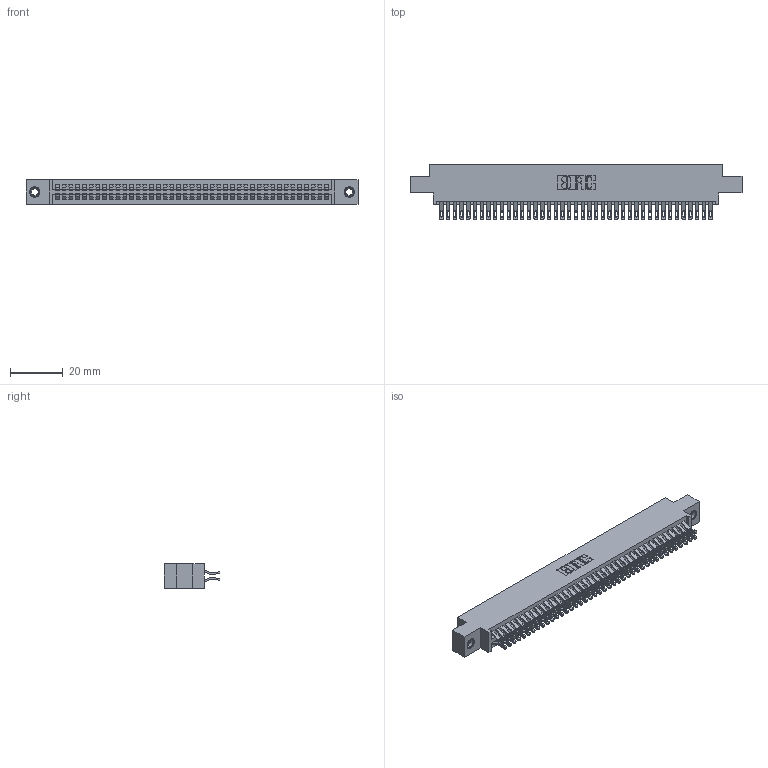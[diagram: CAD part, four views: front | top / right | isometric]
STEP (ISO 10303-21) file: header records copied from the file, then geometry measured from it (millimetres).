
FILE_DESCRIPTION (( 'STEP AP203' ), '1' );
FILE_NAME ('395-082-555-807.STEP', '2019-10-25T07:14:10', ( '' ), ( '' ), 'SwSTEP 2.0', 'SolidWorks 2016', '' );
FILE_SCHEMA (( 'CONFIG_CONTROL_DESIGN' ));
Length unit declared in the file: inch
Products named in the file (4): 345 Part_0.170 Offset - 0.156 Dia-TI; 345-292-001_555 Tail; 345-250-001_345-250-005-103; 395-082-555-807
Assembly tree (85 placements, depth 2):
  395-082-555-807
    345 Part_0.170 Offset - 0.156 Dia-TI
    345-292-001_555 Tail  x82
    345-250-001_345-250-005-103  x2
Bounding box: 125.35 x 21.13 x 9.4 mm (x, y, z)
Volume: 12278.2 mm3; surface area: 19128.5 mm2
Topology: 85 solids, 85 shells, 4782 faces, 15003 edges, 9994 vertices
Faces by surface type: plane 2658, cylinder 2108, cone 12, torus 4
Entity records: 33948 total; most frequent: CARTESIAN_POINT 5709, ORIENTED_EDGE 5606, DIRECTION 5029, EDGE_CURVE 2803, LINE 2467, VECTOR 2467, VERTEX_POINT 1864, AXIS2_PLACEMENT_3D 1281
